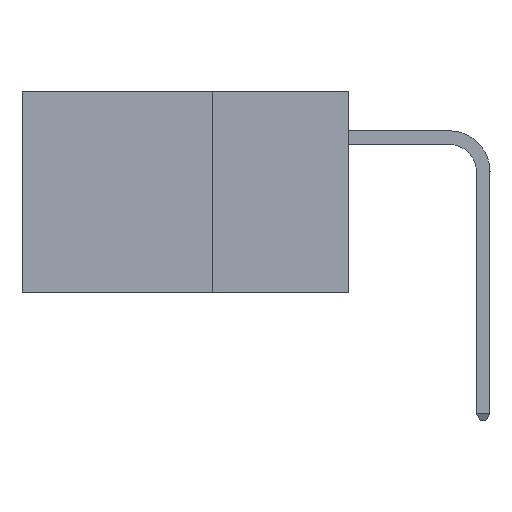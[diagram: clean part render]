
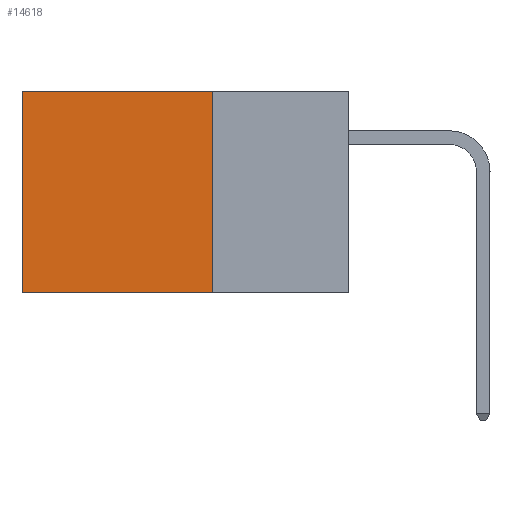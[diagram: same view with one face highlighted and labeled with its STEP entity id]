
A CAD part, left-side view. The second image highlights one B-rep face of the part: STEP entity #14618.
In plain terms, the highlighted planar face has unit normal (-1, 0, 0).
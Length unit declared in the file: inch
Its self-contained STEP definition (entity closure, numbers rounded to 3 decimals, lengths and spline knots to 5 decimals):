
#39 = VECTOR ( 'NONE', #10101, 39.37008 ) ;
#1600 = LINE ( 'NONE', #19917, #39 ) ;
#3966 = DIRECTION ( 'NONE',  ( 0., 1., 0. ) ) ;
#4061 = VERTEX_POINT ( 'NONE', #15274 ) ;
#4826 = EDGE_CURVE ( 'NONE', #20142, #25879, #11786, .T. ) ;
#5066 = VECTOR ( 'NONE', #3966, 39.37008 ) ;
#5158 = DIRECTION ( 'NONE',  ( 0., 0., -1. ) ) ;
#6431 = DIRECTION ( 'NONE',  ( 0., 0., -1. ) ) ;
#6738 = LINE ( 'NONE', #10416, #39844 ) ;
#10101 = DIRECTION ( 'NONE',  ( 0., 0., -1. ) ) ;
#10364 = CARTESIAN_POINT ( 'NONE',  ( 0.2875, 0.25, -0.37 ) ) ;
#10416 = CARTESIAN_POINT ( 'NONE',  ( 0.2875, 0.25, 0. ) ) ;
#11472 = AXIS2_PLACEMENT_3D ( 'NONE', #36519, #13420, #6431 ) ;
#11786 = LINE ( 'NONE', #26338, #5066 ) ;
#13420 = DIRECTION ( 'NONE',  ( 1., 0., 0. ) ) ;
#14618 = ADVANCED_FACE ( 'NONE', ( #39090 ), #20029, .F. ) ;
#14967 = EDGE_CURVE ( 'NONE', #4061, #20142, #21411, .T. ) ;
#15274 = CARTESIAN_POINT ( 'NONE',  ( 0.2875, 0.25, 0. ) ) ;
#17966 = EDGE_CURVE ( 'NONE', #4061, #41514, #6738, .T. ) ;
#18269 = CARTESIAN_POINT ( 'NONE',  ( 0.2875, 0.25, 0. ) ) ;
#19917 = CARTESIAN_POINT ( 'NONE',  ( 0.2875, 0.6, 0. ) ) ;
#20029 = PLANE ( 'NONE',  #11472 ) ;
#20100 = ORIENTED_EDGE ( 'NONE', *, *, #4826, .F. ) ;
#20142 = VERTEX_POINT ( 'NONE', #10364 ) ;
#21411 = LINE ( 'NONE', #18269, #24509 ) ;
#22199 = EDGE_CURVE ( 'NONE', #41514, #25879, #1600, .T. ) ;
#22902 = EDGE_LOOP ( 'NONE', ( #25880, #20100, #35775, #38846 ) ) ;
#24509 = VECTOR ( 'NONE', #5158, 39.37008 ) ;
#25879 = VERTEX_POINT ( 'NONE', #35525 ) ;
#25880 = ORIENTED_EDGE ( 'NONE', *, *, #22199, .T. ) ;
#26338 = CARTESIAN_POINT ( 'NONE',  ( 0.2875, 0.25, -0.37 ) ) ;
#31101 = DIRECTION ( 'NONE',  ( 0., 1., 0. ) ) ;
#35525 = CARTESIAN_POINT ( 'NONE',  ( 0.2875, 0.6, -0.37 ) ) ;
#35775 = ORIENTED_EDGE ( 'NONE', *, *, #14967, .F. ) ;
#36519 = CARTESIAN_POINT ( 'NONE',  ( 0.2875, 0.25, 0. ) ) ;
#36616 = CARTESIAN_POINT ( 'NONE',  ( 0.2875, 0.6, 0. ) ) ;
#38846 = ORIENTED_EDGE ( 'NONE', *, *, #17966, .T. ) ;
#39090 = FACE_OUTER_BOUND ( 'NONE', #22902, .T. ) ;
#39844 = VECTOR ( 'NONE', #31101, 39.37008 ) ;
#41514 = VERTEX_POINT ( 'NONE', #36616 ) ;
